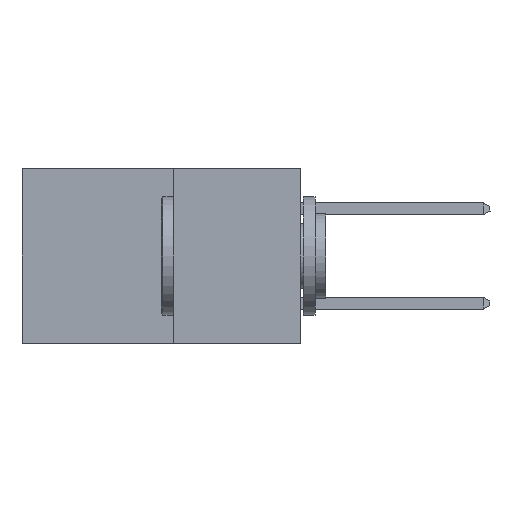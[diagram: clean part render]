
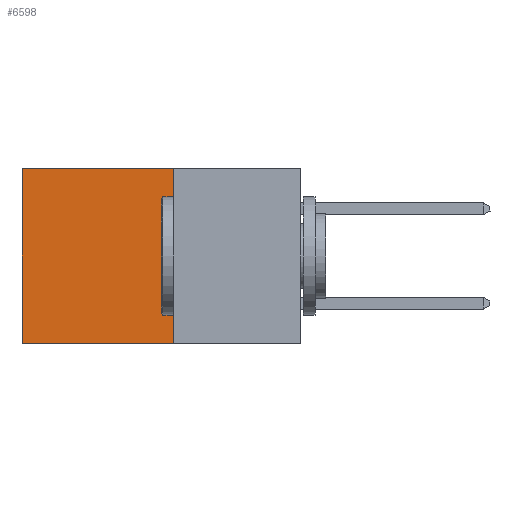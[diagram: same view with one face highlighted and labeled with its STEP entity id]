
A CAD part, left-side view. The second image highlights one B-rep face of the part: STEP entity #6598.
In plain terms, the highlighted planar face has unit normal (-1, 0, 0).
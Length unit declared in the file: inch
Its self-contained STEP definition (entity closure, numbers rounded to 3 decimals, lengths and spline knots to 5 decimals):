
#455 = FACE_OUTER_BOUND ( 'NONE', #8479, .T. ) ;
#1095 = ORIENTED_EDGE ( 'NONE', *, *, #13378, .F. ) ;
#2761 = VERTEX_POINT ( 'NONE', #6035 ) ;
#4079 = VECTOR ( 'NONE', #6835, 39.37008 ) ;
#4565 = VECTOR ( 'NONE', #12249, 39.37008 ) ;
#4795 = DIRECTION ( 'NONE',  ( 0., 0., -1. ) ) ;
#4817 = DIRECTION ( 'NONE',  ( 1., 0., 0. ) ) ;
#4842 = PLANE ( 'NONE',  #14778 ) ;
#4844 = CARTESIAN_POINT ( 'NONE',  ( 0.277, 0.27, -0.37 ) ) ;
#5560 = EDGE_CURVE ( 'NONE', #8703, #14579, #6014, .T. ) ;
#6014 = LINE ( 'NONE', #16691, #12492 ) ;
#6035 = CARTESIAN_POINT ( 'NONE',  ( 0.277, 0.27, 0. ) ) ;
#6067 = LINE ( 'NONE', #8835, #15596 ) ;
#6598 = ADVANCED_FACE ( 'NONE', ( #455 ), #4842, .F. ) ;
#6611 = ORIENTED_EDGE ( 'NONE', *, *, #5560, .T. ) ;
#6835 = DIRECTION ( 'NONE',  ( 0., 1., 0. ) ) ;
#8479 = EDGE_LOOP ( 'NONE', ( #6611, #1095, #14546, #9320 ) ) ;
#8703 = VERTEX_POINT ( 'NONE', #14565 ) ;
#8835 = CARTESIAN_POINT ( 'NONE',  ( 0.277, 0.27, -0.37 ) ) ;
#9320 = ORIENTED_EDGE ( 'NONE', *, *, #11081, .T. ) ;
#9719 = EDGE_CURVE ( 'NONE', #2761, #14317, #6067, .T. ) ;
#10980 = CARTESIAN_POINT ( 'NONE',  ( 0.277, 0.27, 0. ) ) ;
#11019 = LINE ( 'NONE', #11991, #4079 ) ;
#11081 = EDGE_CURVE ( 'NONE', #2761, #8703, #14947, .T. ) ;
#11991 = CARTESIAN_POINT ( 'NONE',  ( 0.277, 0.27, -0.37 ) ) ;
#12249 = DIRECTION ( 'NONE',  ( 0., 1., 0. ) ) ;
#12457 = CARTESIAN_POINT ( 'NONE',  ( 0.277, 0.27, -0.37 ) ) ;
#12492 = VECTOR ( 'NONE', #16721, 39.37008 ) ;
#13378 = EDGE_CURVE ( 'NONE', #14317, #14579, #11019, .T. ) ;
#14317 = VERTEX_POINT ( 'NONE', #12457 ) ;
#14546 = ORIENTED_EDGE ( 'NONE', *, *, #9719, .F. ) ;
#14565 = CARTESIAN_POINT ( 'NONE',  ( 0.277, 0.59, 0. ) ) ;
#14579 = VERTEX_POINT ( 'NONE', #15740 ) ;
#14778 = AXIS2_PLACEMENT_3D ( 'NONE', #4844, #4817, #4795 ) ;
#14947 = LINE ( 'NONE', #10980, #4565 ) ;
#15289 = DIRECTION ( 'NONE',  ( 0., 0., -1. ) ) ;
#15596 = VECTOR ( 'NONE', #15289, 39.37008 ) ;
#15740 = CARTESIAN_POINT ( 'NONE',  ( 0.277, 0.59, -0.37 ) ) ;
#16691 = CARTESIAN_POINT ( 'NONE',  ( 0.277, 0.59, -0.37 ) ) ;
#16721 = DIRECTION ( 'NONE',  ( 0., 0., -1. ) ) ;
